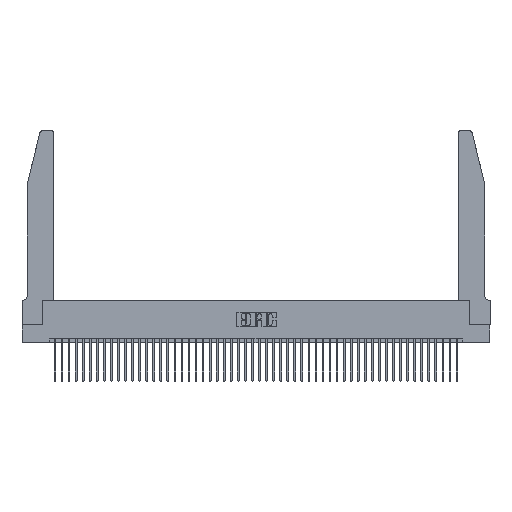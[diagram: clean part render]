
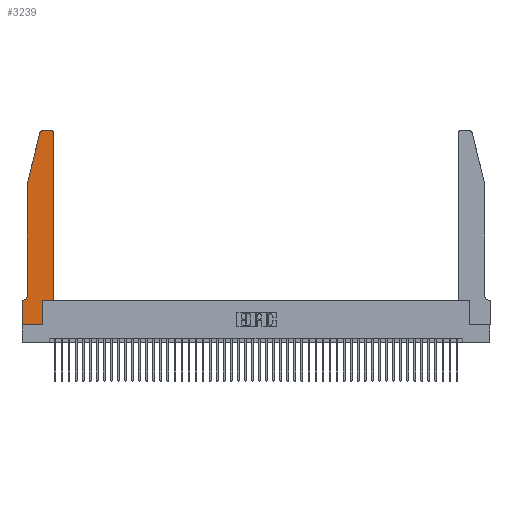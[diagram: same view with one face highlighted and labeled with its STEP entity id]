
A CAD part, top view. The second image highlights one B-rep face of the part: STEP entity #3239.
In plain terms, the highlighted planar face has unit normal (0, 0, 1).
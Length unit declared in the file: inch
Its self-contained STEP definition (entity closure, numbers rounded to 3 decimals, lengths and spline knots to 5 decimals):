
#549 = AXIS2_PLACEMENT_3D ( 'NONE', #20198, #31088, #46198 ) ;
#687 = VERTEX_POINT ( 'NONE', #28024 ) ;
#1383 = ORIENTED_EDGE ( 'NONE', *, *, #24485, .T. ) ;
#1473 = EDGE_LOOP ( 'NONE', ( #37383, #39532, #20617, #18464, #1383, #43092, #3075, #32917, #41661, #45116, #22601, #47303 ) ) ;
#2387 = DIRECTION ( 'NONE',  ( -1., 0., 0. ) ) ;
#3075 = ORIENTED_EDGE ( 'NONE', *, *, #43879, .T. ) ;
#3239 = ADVANCED_FACE ( 'NONE', ( #29141 ), #38077, .T. ) ;
#4291 = CARTESIAN_POINT ( 'NONE',  ( 0.284, 2.72, 0.37 ) ) ;
#4724 = CARTESIAN_POINT ( 'NONE',  ( 0., 0.35, 0.37 ) ) ;
#4848 = DIRECTION ( 'NONE',  ( 0., 0., -1. ) ) ;
#5033 = AXIS2_PLACEMENT_3D ( 'NONE', #4724, #45344, #12540 ) ;
#5174 = VERTEX_POINT ( 'NONE', #20647 ) ;
#5496 = VERTEX_POINT ( 'NONE', #13242 ) ;
#6213 = DIRECTION ( 'NONE',  ( -1., 0., 0. ) ) ;
#6582 = CARTESIAN_POINT ( 'NONE',  ( 0.0755, 2., 0.37 ) ) ;
#7998 = EDGE_CURVE ( 'NONE', #43145, #37882, #13077, .T. ) ;
#8141 = DIRECTION ( 'NONE',  ( 0., 1., 0. ) ) ;
#8482 = EDGE_CURVE ( 'NONE', #687, #47017, #39768, .T. ) ;
#10327 = DIRECTION ( 'NONE',  ( -0.239, -0.971, 0. ) ) ;
#10582 = VECTOR ( 'NONE', #8141, 39.37008 ) ;
#11416 = VECTOR ( 'NONE', #47967, 39.37008 ) ;
#11516 = EDGE_CURVE ( 'NONE', #5174, #43145, #32539, .T. ) ;
#12050 = VECTOR ( 'NONE', #15218, 39.37008 ) ;
#12540 = DIRECTION ( 'NONE',  ( 1., 0., 0. ) ) ;
#12808 = DIRECTION ( 'NONE',  ( 0., -1., 0. ) ) ;
#13077 = LINE ( 'NONE', #39548, #19441 ) ;
#13242 = CARTESIAN_POINT ( 'NONE',  ( 0.4505, 0.35, 0.37 ) ) ;
#14535 = EDGE_CURVE ( 'NONE', #5496, #5174, #45423, .T. ) ;
#15218 = DIRECTION ( 'NONE',  ( 0., 1., 0. ) ) ;
#16538 = DIRECTION ( 'NONE',  ( 1., 0., 0. ) ) ;
#17062 = VECTOR ( 'NONE', #16538, 39.37008 ) ;
#18455 = VECTOR ( 'NONE', #10327, 39.37008 ) ;
#18464 = ORIENTED_EDGE ( 'NONE', *, *, #37468, .T. ) ;
#18914 = DIRECTION ( 'NONE',  ( 1., 0., 0. ) ) ;
#19172 = CARTESIAN_POINT ( 'NONE',  ( 0.4505, 0.35, 0.37 ) ) ;
#19441 = VECTOR ( 'NONE', #6213, 39.37008 ) ;
#19796 = DIRECTION ( 'NONE',  ( -1., 0., 0. ) ) ;
#20198 = CARTESIAN_POINT ( 'NONE',  ( 0.4205, 2.72, 0.37 ) ) ;
#20492 = CIRCLE ( 'NONE', #33698, 0.07 ) ;
#20617 = ORIENTED_EDGE ( 'NONE', *, *, #25430, .T. ) ;
#20647 = CARTESIAN_POINT ( 'NONE',  ( 0.4505, 2.72, 0.37 ) ) ;
#20776 = CARTESIAN_POINT ( 'NONE',  ( 0.25487, 2.72718, 0.37 ) ) ;
#21886 = LINE ( 'NONE', #41425, #12050 ) ;
#22419 = EDGE_CURVE ( 'NONE', #43932, #5496, #32912, .T. ) ;
#22497 = DIRECTION ( 'NONE',  ( 0., 0., 1. ) ) ;
#22601 = ORIENTED_EDGE ( 'NONE', *, *, #14535, .T. ) ;
#23924 = VECTOR ( 'NONE', #34994, 39.37008 ) ;
#24230 = CARTESIAN_POINT ( 'NONE',  ( 0., 0., 0.37 ) ) ;
#24485 = EDGE_CURVE ( 'NONE', #45528, #31258, #20492, .T. ) ;
#25430 = EDGE_CURVE ( 'NONE', #48052, #47027, #38269, .T. ) ;
#25522 = CARTESIAN_POINT ( 'NONE',  ( 0., 0.35, 0.37 ) ) ;
#27478 = VECTOR ( 'NONE', #12808, 39.37008 ) ;
#28024 = CARTESIAN_POINT ( 'NONE',  ( 0., 0., 0.37 ) ) ;
#28928 = CARTESIAN_POINT ( 'NONE',  ( 0.4505, 0.35, 0.37 ) ) ;
#29141 = FACE_OUTER_BOUND ( 'NONE', #1473, .T. ) ;
#29723 = CARTESIAN_POINT ( 'NONE',  ( 0.2865, 0., 0.37 ) ) ;
#29776 = EDGE_CURVE ( 'NONE', #47017, #43932, #21886, .T. ) ;
#30216 = CARTESIAN_POINT ( 'NONE',  ( 0.0055, 0.42, 0.37 ) ) ;
#30227 = CARTESIAN_POINT ( 'NONE',  ( 0.0055, 0.35, 0.37 ) ) ;
#31088 = DIRECTION ( 'NONE',  ( 0., 0., 1. ) ) ;
#31258 = VERTEX_POINT ( 'NONE', #30227 ) ;
#31578 = CIRCLE ( 'NONE', #47196, 0.03 ) ;
#32139 = EDGE_CURVE ( 'NONE', #31258, #44174, #38739, .T. ) ;
#32539 = CIRCLE ( 'NONE', #549, 0.03 ) ;
#32683 = LINE ( 'NONE', #24230, #23924 ) ;
#32912 = LINE ( 'NONE', #28928, #11416 ) ;
#32917 = ORIENTED_EDGE ( 'NONE', *, *, #8482, .T. ) ;
#32961 = CARTESIAN_POINT ( 'NONE',  ( 0.0755, 0.42, 0.37 ) ) ;
#33698 = AXIS2_PLACEMENT_3D ( 'NONE', #30216, #4848, #19796 ) ;
#34994 = DIRECTION ( 'NONE',  ( 0., -1., 0. ) ) ;
#37383 = ORIENTED_EDGE ( 'NONE', *, *, #7998, .T. ) ;
#37468 = EDGE_CURVE ( 'NONE', #47027, #45528, #40396, .T. ) ;
#37474 = CARTESIAN_POINT ( 'NONE',  ( 0.284, 2.75, 0.37 ) ) ;
#37847 = EDGE_CURVE ( 'NONE', #37882, #48052, #31578, .T. ) ;
#37882 = VERTEX_POINT ( 'NONE', #37474 ) ;
#38077 = PLANE ( 'NONE',  #5033 ) ;
#38269 = LINE ( 'NONE', #6582, #18455 ) ;
#38683 = CARTESIAN_POINT ( 'NONE',  ( 0., 0., 0.37 ) ) ;
#38739 = LINE ( 'NONE', #39627, #39335 ) ;
#39335 = VECTOR ( 'NONE', #2387, 39.37008 ) ;
#39532 = ORIENTED_EDGE ( 'NONE', *, *, #37847, .T. ) ;
#39548 = CARTESIAN_POINT ( 'NONE',  ( 0.2605, 2.75, 0.37 ) ) ;
#39627 = CARTESIAN_POINT ( 'NONE',  ( 0.0755, 0.35, 0.37 ) ) ;
#39768 = LINE ( 'NONE', #38683, #17062 ) ;
#40396 = LINE ( 'NONE', #42738, #27478 ) ;
#41425 = CARTESIAN_POINT ( 'NONE',  ( 0.2865, 0.35, 0.37 ) ) ;
#41661 = ORIENTED_EDGE ( 'NONE', *, *, #29776, .T. ) ;
#41874 = CARTESIAN_POINT ( 'NONE',  ( 0.4205, 2.75, 0.37 ) ) ;
#42738 = CARTESIAN_POINT ( 'NONE',  ( 0.0755, 2., 0.37 ) ) ;
#43092 = ORIENTED_EDGE ( 'NONE', *, *, #32139, .T. ) ;
#43145 = VERTEX_POINT ( 'NONE', #41874 ) ;
#43879 = EDGE_CURVE ( 'NONE', #44174, #687, #32683, .T. ) ;
#43932 = VERTEX_POINT ( 'NONE', #46687 ) ;
#44174 = VERTEX_POINT ( 'NONE', #25522 ) ;
#45116 = ORIENTED_EDGE ( 'NONE', *, *, #22419, .T. ) ;
#45344 = DIRECTION ( 'NONE',  ( 0., 0., 1. ) ) ;
#45423 = LINE ( 'NONE', #19172, #10582 ) ;
#45528 = VERTEX_POINT ( 'NONE', #32961 ) ;
#46198 = DIRECTION ( 'NONE',  ( 1., 0., 0. ) ) ;
#46687 = CARTESIAN_POINT ( 'NONE',  ( 0.2865, 0.35, 0.37 ) ) ;
#47017 = VERTEX_POINT ( 'NONE', #29723 ) ;
#47027 = VERTEX_POINT ( 'NONE', #47961 ) ;
#47196 = AXIS2_PLACEMENT_3D ( 'NONE', #4291, #22497, #18914 ) ;
#47303 = ORIENTED_EDGE ( 'NONE', *, *, #11516, .T. ) ;
#47961 = CARTESIAN_POINT ( 'NONE',  ( 0.0755, 2., 0.37 ) ) ;
#47967 = DIRECTION ( 'NONE',  ( 1., 0., 0. ) ) ;
#48052 = VERTEX_POINT ( 'NONE', #20776 ) ;
